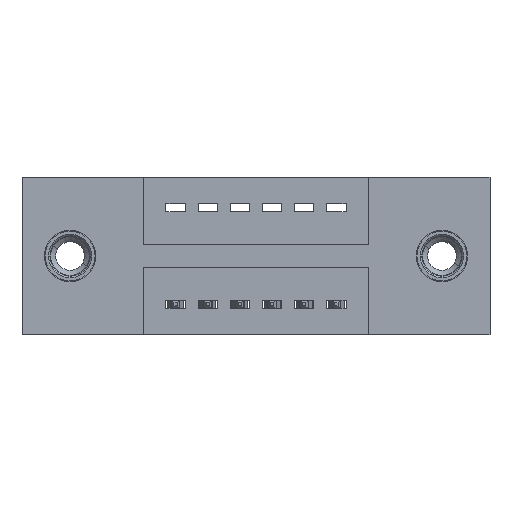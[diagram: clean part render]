
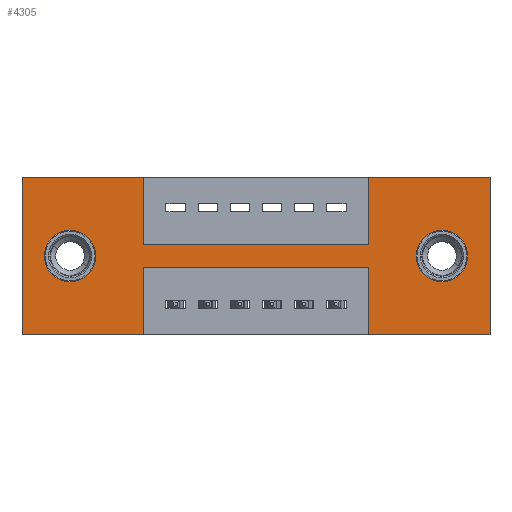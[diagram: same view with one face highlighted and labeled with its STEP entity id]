
A CAD part, front view. The second image highlights one B-rep face of the part: STEP entity #4305.
In plain terms, the highlighted planar face has unit normal (0, -1, 0).
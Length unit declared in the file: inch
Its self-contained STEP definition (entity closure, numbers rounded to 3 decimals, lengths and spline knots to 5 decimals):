
#56 = ORIENTED_EDGE ( 'NONE', *, *, #9238, .T. ) ;
#147 = CARTESIAN_POINT ( 'NONE',  ( 1.455, 0., 0. ) ) ;
#166 = VECTOR ( 'NONE', #3295, 39.37008 ) ;
#440 = CARTESIAN_POINT ( 'NONE',  ( 0., 0., -0.49 ) ) ;
#441 = VERTEX_POINT ( 'NONE', #4867 ) ;
#457 = DIRECTION ( 'NONE',  ( -1., 0., 0. ) ) ;
#681 = AXIS2_PLACEMENT_3D ( 'NONE', #2521, #1085, #1829 ) ;
#693 = VECTOR ( 'NONE', #4124, 39.37008 ) ;
#752 = AXIS2_PLACEMENT_3D ( 'NONE', #4572, #8210, #1568 ) ;
#772 = VERTEX_POINT ( 'NONE', #3625 ) ;
#851 = LINE ( 'NONE', #3937, #166 ) ;
#930 = LINE ( 'NONE', #2647, #693 ) ;
#968 = VERTEX_POINT ( 'NONE', #147 ) ;
#1070 = EDGE_CURVE ( 'NONE', #5856, #3929, #4152, .T. ) ;
#1071 = EDGE_CURVE ( 'NONE', #2275, #968, #6135, .T. ) ;
#1074 = DIRECTION ( 'NONE',  ( 0., 0., -1. ) ) ;
#1085 = DIRECTION ( 'NONE',  ( 0., 1., 0. ) ) ;
#1092 = DIRECTION ( 'NONE',  ( 0., 0., 1. ) ) ;
#1339 = LINE ( 'NONE', #8950, #7827 ) ;
#1411 = VERTEX_POINT ( 'NONE', #4067 ) ;
#1448 = DIRECTION ( 'NONE',  ( 0., 0., 1. ) ) ;
#1568 = DIRECTION ( 'NONE',  ( 0., 0., -1. ) ) ;
#1606 = CARTESIAN_POINT ( 'NONE',  ( 0., 0., 0. ) ) ;
#1646 = DIRECTION ( 'NONE',  ( 0., 0., -1. ) ) ;
#1648 = ORIENTED_EDGE ( 'NONE', *, *, #1070, .T. ) ;
#1753 = CARTESIAN_POINT ( 'NONE',  ( 0.1495, 0., -0.165 ) ) ;
#1829 = DIRECTION ( 'NONE',  ( 0., 0., 1. ) ) ;
#1831 = VERTEX_POINT ( 'NONE', #2468 ) ;
#1857 = CARTESIAN_POINT ( 'NONE',  ( 0.3775, 0., -0.49 ) ) ;
#1871 = VECTOR ( 'NONE', #8002, 39.37008 ) ;
#1948 = FACE_BOUND ( 'NONE', #7908, .T. ) ;
#1983 = DIRECTION ( 'NONE',  ( 0., 0., 1. ) ) ;
#2076 = DIRECTION ( 'NONE',  ( 0., 0., -1. ) ) ;
#2135 = VECTOR ( 'NONE', #1092, 39.37008 ) ;
#2240 = LINE ( 'NONE', #6938, #7300 ) ;
#2275 = VERTEX_POINT ( 'NONE', #3877 ) ;
#2285 = LINE ( 'NONE', #8735, #7820 ) ;
#2309 = EDGE_CURVE ( 'NONE', #5998, #441, #4076, .T. ) ;
#2310 = EDGE_CURVE ( 'NONE', #968, #9331, #851, .T. ) ;
#2312 = VERTEX_POINT ( 'NONE', #1857 ) ;
#2337 = EDGE_CURVE ( 'NONE', #772, #1831, #2240, .T. ) ;
#2377 = DIRECTION ( 'NONE',  ( 1., 0., 0. ) ) ;
#2453 = LINE ( 'NONE', #4425, #3367 ) ;
#2468 = CARTESIAN_POINT ( 'NONE',  ( 0.3775, 0., -0.28 ) ) ;
#2521 = CARTESIAN_POINT ( 'NONE',  ( 0.1495, 0., -0.245 ) ) ;
#2524 = DIRECTION ( 'NONE',  ( -1., 0., 0. ) ) ;
#2540 = VERTEX_POINT ( 'NONE', #6438 ) ;
#2597 = AXIS2_PLACEMENT_3D ( 'NONE', #9457, #7240, #1983 ) ;
#2602 = DIRECTION ( 'NONE',  ( 0., 1., 0. ) ) ;
#2647 = CARTESIAN_POINT ( 'NONE',  ( 0.3775, 0., -0.28 ) ) ;
#2821 = EDGE_CURVE ( 'NONE', #3134, #6988, #5799, .T. ) ;
#2858 = ORIENTED_EDGE ( 'NONE', *, *, #6167, .F. ) ;
#2867 = EDGE_CURVE ( 'NONE', #6988, #5998, #6596, .T. ) ;
#2890 = CARTESIAN_POINT ( 'NONE',  ( 1.3055, 0., -0.165 ) ) ;
#2894 = VECTOR ( 'NONE', #457, 39.37008 ) ;
#3134 = VERTEX_POINT ( 'NONE', #440 ) ;
#3230 = CARTESIAN_POINT ( 'NONE',  ( 0., 0., -0.49 ) ) ;
#3241 = CARTESIAN_POINT ( 'NONE',  ( 1.0775, 0., -0.28 ) ) ;
#3295 = DIRECTION ( 'NONE',  ( 0., 0., -1. ) ) ;
#3350 = FACE_OUTER_BOUND ( 'NONE', #5475, .T. ) ;
#3367 = VECTOR ( 'NONE', #1448, 39.37008 ) ;
#3421 = EDGE_CURVE ( 'NONE', #7330, #2275, #2453, .T. ) ;
#3424 = VERTEX_POINT ( 'NONE', #2890 ) ;
#3517 = CARTESIAN_POINT ( 'NONE',  ( 0., 0., 0. ) ) ;
#3625 = CARTESIAN_POINT ( 'NONE',  ( 1.0775, 0., -0.28 ) ) ;
#3691 = CARTESIAN_POINT ( 'NONE',  ( 1.455, 0., -0.49 ) ) ;
#3877 = CARTESIAN_POINT ( 'NONE',  ( 1.0775, 0., 0. ) ) ;
#3881 = EDGE_CURVE ( 'NONE', #1831, #2312, #930, .T. ) ;
#3906 = EDGE_LOOP ( 'NONE', ( #1648, #8561 ) ) ;
#3929 = VERTEX_POINT ( 'NONE', #7953 ) ;
#3937 = CARTESIAN_POINT ( 'NONE',  ( 1.455, 0., 0. ) ) ;
#4067 = CARTESIAN_POINT ( 'NONE',  ( 1.0775, 0., -0.49 ) ) ;
#4076 = LINE ( 'NONE', #4507, #8685 ) ;
#4124 = DIRECTION ( 'NONE',  ( 0., 0., -1. ) ) ;
#4152 = CIRCLE ( 'NONE', #2597, 0.08 ) ;
#4238 = DIRECTION ( 'NONE',  ( 1., 0., 0. ) ) ;
#4305 = ADVANCED_FACE ( 'NONE', ( #1948, #6572, #3350 ), #8147, .T. ) ;
#4308 = CIRCLE ( 'NONE', #681, 0.08 ) ;
#4320 = AXIS2_PLACEMENT_3D ( 'NONE', #4839, #2602, #1074 ) ;
#4416 = EDGE_CURVE ( 'NONE', #2312, #3134, #7839, .T. ) ;
#4425 = CARTESIAN_POINT ( 'NONE',  ( 1.0775, 0., -0.21 ) ) ;
#4437 = DIRECTION ( 'NONE',  ( 0., 0., 1. ) ) ;
#4507 = CARTESIAN_POINT ( 'NONE',  ( 0.3775, 0., -0.21 ) ) ;
#4572 = CARTESIAN_POINT ( 'NONE',  ( 0., 0., -0.49 ) ) ;
#4666 = ORIENTED_EDGE ( 'NONE', *, *, #8325, .F. ) ;
#4839 = CARTESIAN_POINT ( 'NONE',  ( 1.3055, 0., -0.245 ) ) ;
#4867 = CARTESIAN_POINT ( 'NONE',  ( 0.3775, 0., -0.21 ) ) ;
#5000 = CARTESIAN_POINT ( 'NONE',  ( 0.3775, 0., 0. ) ) ;
#5123 = ORIENTED_EDGE ( 'NONE', *, *, #4416, .F. ) ;
#5475 = EDGE_LOOP ( 'NONE', ( #8469, #8858, #7079, #6617, #7231, #5123, #8960, #6445, #4666, #2858, #9372, #7982 ) ) ;
#5595 = CIRCLE ( 'NONE', #7965, 0.08 ) ;
#5699 = EDGE_CURVE ( 'NONE', #441, #7330, #1339, .T. ) ;
#5799 = LINE ( 'NONE', #6634, #8339 ) ;
#5817 = CIRCLE ( 'NONE', #4320, 0.08 ) ;
#5856 = VERTEX_POINT ( 'NONE', #1753 ) ;
#5883 = DIRECTION ( 'NONE',  ( -1., 0., 0. ) ) ;
#5998 = VERTEX_POINT ( 'NONE', #5000 ) ;
#6135 = LINE ( 'NONE', #8652, #8320 ) ;
#6167 = EDGE_CURVE ( 'NONE', #9331, #1411, #2285, .T. ) ;
#6438 = CARTESIAN_POINT ( 'NONE',  ( 1.3055, 0., -0.325 ) ) ;
#6445 = ORIENTED_EDGE ( 'NONE', *, *, #2337, .F. ) ;
#6530 = CARTESIAN_POINT ( 'NONE',  ( 1.0775, 0., -0.21 ) ) ;
#6572 = FACE_BOUND ( 'NONE', #3906, .T. ) ;
#6596 = LINE ( 'NONE', #3517, #1871 ) ;
#6617 = ORIENTED_EDGE ( 'NONE', *, *, #2867, .F. ) ;
#6634 = CARTESIAN_POINT ( 'NONE',  ( 0., 0., 0. ) ) ;
#6938 = CARTESIAN_POINT ( 'NONE',  ( 0.3775, 0., -0.28 ) ) ;
#6988 = VERTEX_POINT ( 'NONE', #1606 ) ;
#7079 = ORIENTED_EDGE ( 'NONE', *, *, #2309, .F. ) ;
#7231 = ORIENTED_EDGE ( 'NONE', *, *, #2821, .F. ) ;
#7240 = DIRECTION ( 'NONE',  ( 0., 1., 0. ) ) ;
#7300 = VECTOR ( 'NONE', #2524, 39.37008 ) ;
#7330 = VERTEX_POINT ( 'NONE', #6530 ) ;
#7334 = DIRECTION ( 'NONE',  ( 0., 1., 0. ) ) ;
#7820 = VECTOR ( 'NONE', #5883, 39.37008 ) ;
#7827 = VECTOR ( 'NONE', #2377, 39.37008 ) ;
#7839 = LINE ( 'NONE', #3230, #2894 ) ;
#7908 = EDGE_LOOP ( 'NONE', ( #56, #8819 ) ) ;
#7953 = CARTESIAN_POINT ( 'NONE',  ( 0.1495, 0., -0.325 ) ) ;
#7965 = AXIS2_PLACEMENT_3D ( 'NONE', #8011, #7334, #2076 ) ;
#7982 = ORIENTED_EDGE ( 'NONE', *, *, #1071, .F. ) ;
#8002 = DIRECTION ( 'NONE',  ( 1., 0., 0. ) ) ;
#8011 = CARTESIAN_POINT ( 'NONE',  ( 1.3055, 0., -0.245 ) ) ;
#8147 = PLANE ( 'NONE',  #752 ) ;
#8210 = DIRECTION ( 'NONE',  ( 0., -1., 0. ) ) ;
#8320 = VECTOR ( 'NONE', #4238, 39.37008 ) ;
#8325 = EDGE_CURVE ( 'NONE', #1411, #772, #8707, .T. ) ;
#8339 = VECTOR ( 'NONE', #4437, 39.37008 ) ;
#8469 = ORIENTED_EDGE ( 'NONE', *, *, #3421, .F. ) ;
#8561 = ORIENTED_EDGE ( 'NONE', *, *, #8932, .T. ) ;
#8652 = CARTESIAN_POINT ( 'NONE',  ( 0., 0., 0. ) ) ;
#8685 = VECTOR ( 'NONE', #1646, 39.37008 ) ;
#8707 = LINE ( 'NONE', #3241, #2135 ) ;
#8735 = CARTESIAN_POINT ( 'NONE',  ( 0., 0., -0.49 ) ) ;
#8819 = ORIENTED_EDGE ( 'NONE', *, *, #9523, .T. ) ;
#8858 = ORIENTED_EDGE ( 'NONE', *, *, #5699, .F. ) ;
#8932 = EDGE_CURVE ( 'NONE', #3929, #5856, #4308, .T. ) ;
#8950 = CARTESIAN_POINT ( 'NONE',  ( 0.3775, 0., -0.21 ) ) ;
#8960 = ORIENTED_EDGE ( 'NONE', *, *, #3881, .F. ) ;
#9238 = EDGE_CURVE ( 'NONE', #3424, #2540, #5595, .T. ) ;
#9331 = VERTEX_POINT ( 'NONE', #3691 ) ;
#9372 = ORIENTED_EDGE ( 'NONE', *, *, #2310, .F. ) ;
#9457 = CARTESIAN_POINT ( 'NONE',  ( 0.1495, 0., -0.245 ) ) ;
#9523 = EDGE_CURVE ( 'NONE', #2540, #3424, #5817, .T. ) ;
